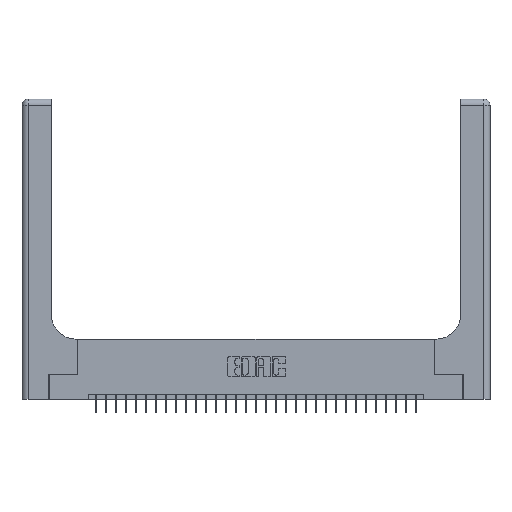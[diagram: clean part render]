
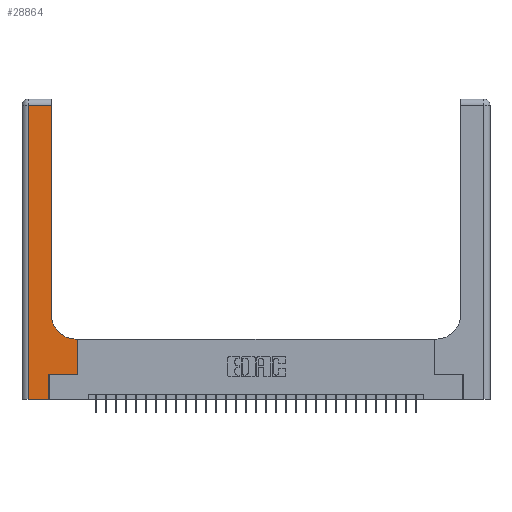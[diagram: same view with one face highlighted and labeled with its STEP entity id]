
A CAD part, top view. The second image highlights one B-rep face of the part: STEP entity #28864.
In plain terms, the highlighted planar face has unit normal (0, 0, 1).
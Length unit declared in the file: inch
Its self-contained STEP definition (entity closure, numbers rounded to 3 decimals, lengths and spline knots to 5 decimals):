
#135 = VECTOR ( 'NONE', #31177, 39.37008 ) ;
#187 = EDGE_CURVE ( 'NONE', #5116, #1387, #8518, .T. ) ;
#1269 = ORIENTED_EDGE ( 'NONE', *, *, #5895, .T. ) ;
#1387 = VERTEX_POINT ( 'NONE', #22947 ) ;
#1413 = DIRECTION ( 'NONE',  ( -1., 0., 0. ) ) ;
#2617 = DIRECTION ( 'NONE',  ( -1., 0., 0. ) ) ;
#2956 = VERTEX_POINT ( 'NONE', #30914 ) ;
#2988 = CARTESIAN_POINT ( 'NONE',  ( 0., 2.94, 0.37 ) ) ;
#3403 = ORIENTED_EDGE ( 'NONE', *, *, #27188, .T. ) ;
#4388 = ORIENTED_EDGE ( 'NONE', *, *, #27960, .T. ) ;
#5042 = VERTEX_POINT ( 'NONE', #23453 ) ;
#5104 = VECTOR ( 'NONE', #30610, 39.37008 ) ;
#5116 = VERTEX_POINT ( 'NONE', #16559 ) ;
#5210 = EDGE_LOOP ( 'NONE', ( #24763, #15852, #9315, #13071, #25404, #3403, #4388, #16749, #1269 ) ) ;
#5895 = EDGE_CURVE ( 'NONE', #2956, #29354, #21549, .T. ) ;
#6159 = DIRECTION ( 'NONE',  ( 0., 0., -1. ) ) ;
#6680 = AXIS2_PLACEMENT_3D ( 'NONE', #10463, #6159, #1413 ) ;
#7144 = VECTOR ( 'NONE', #2617, 39.37008 ) ;
#7196 = DIRECTION ( 'NONE',  ( 0., -1., 0. ) ) ;
#7542 = CARTESIAN_POINT ( 'NONE',  ( 0.2915, 0.6, 0.37 ) ) ;
#7864 = CARTESIAN_POINT ( 'NONE',  ( 0., 0., 0.37 ) ) ;
#8077 = LINE ( 'NONE', #2988, #21066 ) ;
#8518 = LINE ( 'NONE', #22937, #12935 ) ;
#9017 = AXIS2_PLACEMENT_3D ( 'NONE', #22259, #29805, #12130 ) ;
#9250 = VECTOR ( 'NONE', #27678, 39.37008 ) ;
#9315 = ORIENTED_EDGE ( 'NONE', *, *, #31590, .T. ) ;
#10463 = CARTESIAN_POINT ( 'NONE',  ( 0., 3., 0.37 ) ) ;
#10917 = EDGE_CURVE ( 'NONE', #30474, #5042, #8077, .T. ) ;
#11011 = EDGE_CURVE ( 'NONE', #29354, #30474, #24283, .T. ) ;
#12130 = DIRECTION ( 'NONE',  ( 1., 0., 0. ) ) ;
#12340 = CARTESIAN_POINT ( 'NONE',  ( 0.5585, 0.25, 0.37 ) ) ;
#12415 = LINE ( 'NONE', #27167, #21964 ) ;
#12935 = VECTOR ( 'NONE', #18521, 39.37008 ) ;
#12981 = DIRECTION ( 'NONE',  ( -1., 0., 0. ) ) ;
#13071 = ORIENTED_EDGE ( 'NONE', *, *, #17494, .T. ) ;
#14969 = LINE ( 'NONE', #12340, #24532 ) ;
#15852 = ORIENTED_EDGE ( 'NONE', *, *, #10917, .T. ) ;
#16559 = CARTESIAN_POINT ( 'NONE',  ( 0.269, 0., 0.37 ) ) ;
#16664 = VERTEX_POINT ( 'NONE', #21678 ) ;
#16749 = ORIENTED_EDGE ( 'NONE', *, *, #17492, .T. ) ;
#17492 = EDGE_CURVE ( 'NONE', #23997, #2956, #22606, .T. ) ;
#17494 = EDGE_CURVE ( 'NONE', #31622, #5116, #23091, .T. ) ;
#18158 = LINE ( 'NONE', #23078, #5104 ) ;
#18521 = DIRECTION ( 'NONE',  ( 0., 1., 0. ) ) ;
#19886 = DIRECTION ( 'NONE',  ( 0., 1., 0. ) ) ;
#21066 = VECTOR ( 'NONE', #12981, 39.37008 ) ;
#21549 = CIRCLE ( 'NONE', #9017, 0.25 ) ;
#21678 = CARTESIAN_POINT ( 'NONE',  ( 0.5585, 0.25, 0.37 ) ) ;
#21964 = VECTOR ( 'NONE', #7196, 39.37008 ) ;
#22259 = CARTESIAN_POINT ( 'NONE',  ( 0.5415, 0.85, 0.37 ) ) ;
#22606 = LINE ( 'NONE', #7542, #7144 ) ;
#22610 = CARTESIAN_POINT ( 'NONE',  ( 0.5585, 0.6, 0.37 ) ) ;
#22937 = CARTESIAN_POINT ( 'NONE',  ( 0.269, 0., 0.37 ) ) ;
#22947 = CARTESIAN_POINT ( 'NONE',  ( 0.269, 0.25, 0.37 ) ) ;
#23078 = CARTESIAN_POINT ( 'NONE',  ( 0.269, 0.25, 0.37 ) ) ;
#23091 = LINE ( 'NONE', #7864, #9250 ) ;
#23453 = CARTESIAN_POINT ( 'NONE',  ( 0.06, 2.94, 0.37 ) ) ;
#23701 = PLANE ( 'NONE',  #6680 ) ;
#23856 = FACE_OUTER_BOUND ( 'NONE', #5210, .T. ) ;
#23997 = VERTEX_POINT ( 'NONE', #22610 ) ;
#24247 = CARTESIAN_POINT ( 'NONE',  ( 0.06, 0., 0.37 ) ) ;
#24283 = LINE ( 'NONE', #31514, #135 ) ;
#24532 = VECTOR ( 'NONE', #19886, 39.37008 ) ;
#24763 = ORIENTED_EDGE ( 'NONE', *, *, #11011, .T. ) ;
#24873 = CARTESIAN_POINT ( 'NONE',  ( 0.2915, 2.94, 0.37 ) ) ;
#25404 = ORIENTED_EDGE ( 'NONE', *, *, #187, .T. ) ;
#27167 = CARTESIAN_POINT ( 'NONE',  ( 0.06, 3., 0.37 ) ) ;
#27188 = EDGE_CURVE ( 'NONE', #1387, #16664, #18158, .T. ) ;
#27678 = DIRECTION ( 'NONE',  ( 1., 0., 0. ) ) ;
#27960 = EDGE_CURVE ( 'NONE', #16664, #23997, #14969, .T. ) ;
#28864 = ADVANCED_FACE ( 'NONE', ( #23856 ), #23701, .F. ) ;
#29354 = VERTEX_POINT ( 'NONE', #31530 ) ;
#29805 = DIRECTION ( 'NONE',  ( 0., 0., -1. ) ) ;
#30474 = VERTEX_POINT ( 'NONE', #24873 ) ;
#30610 = DIRECTION ( 'NONE',  ( 1., 0., 0. ) ) ;
#30914 = CARTESIAN_POINT ( 'NONE',  ( 0.5415, 0.6, 0.37 ) ) ;
#31177 = DIRECTION ( 'NONE',  ( 0., 1., 0. ) ) ;
#31514 = CARTESIAN_POINT ( 'NONE',  ( 0.2915, 3., 0.37 ) ) ;
#31530 = CARTESIAN_POINT ( 'NONE',  ( 0.2915, 0.85, 0.37 ) ) ;
#31590 = EDGE_CURVE ( 'NONE', #5042, #31622, #12415, .T. ) ;
#31622 = VERTEX_POINT ( 'NONE', #24247 ) ;
